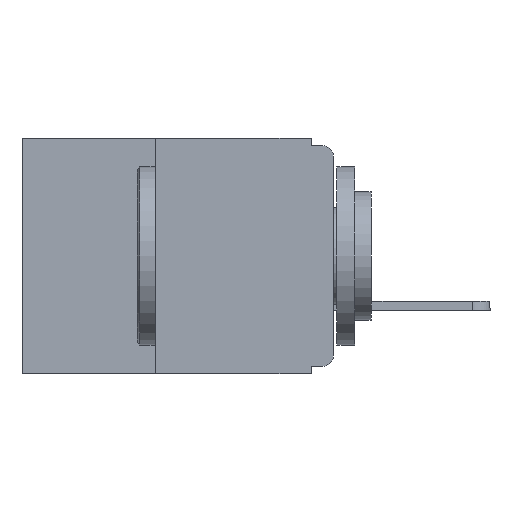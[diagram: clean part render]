
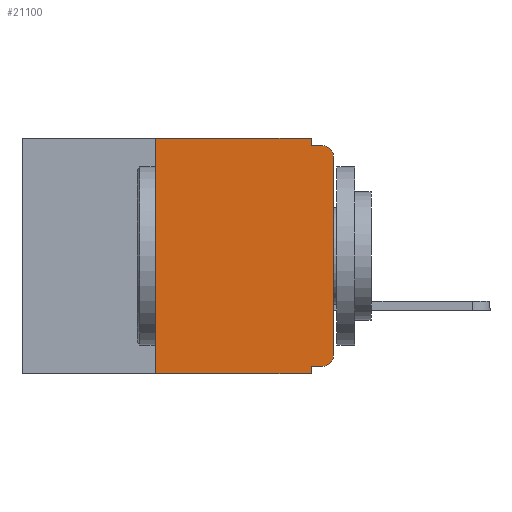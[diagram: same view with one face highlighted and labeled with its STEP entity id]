
A CAD part, left-side view. The second image highlights one B-rep face of the part: STEP entity #21100.
In plain terms, the highlighted planar face has unit normal (-1, 0, 0).
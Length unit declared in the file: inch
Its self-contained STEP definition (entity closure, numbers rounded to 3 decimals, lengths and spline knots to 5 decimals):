
#41 = VECTOR ( 'NONE', #14605, 39.37008 ) ;
#57 = DIRECTION ( 'NONE',  ( 0., -1., 0. ) ) ;
#249 = CARTESIAN_POINT ( 'NONE',  ( 0., 0., 0. ) ) ;
#356 = EDGE_CURVE ( 'NONE', #25342, #8186, #9317, .T. ) ;
#1003 = DIRECTION ( 'NONE',  ( -1., 0., 0. ) ) ;
#1020 = EDGE_CURVE ( 'NONE', #1346, #8186, #3463, .T. ) ;
#1124 = DIRECTION ( 'NONE',  ( -1., 0., 0. ) ) ;
#1240 = ORIENTED_EDGE ( 'NONE', *, *, #22163, .T. ) ;
#1346 = VERTEX_POINT ( 'NONE', #16855 ) ;
#1352 = VECTOR ( 'NONE', #9308, 39.37008 ) ;
#1428 = VERTEX_POINT ( 'NONE', #7016 ) ;
#1798 = VECTOR ( 'NONE', #15691, 39.37008 ) ;
#2524 = CARTESIAN_POINT ( 'NONE',  ( 0., 0., -0.32 ) ) ;
#3062 = PLANE ( 'NONE',  #16985 ) ;
#3365 = CARTESIAN_POINT ( 'NONE',  ( 0., 0.031, -0.33 ) ) ;
#3463 = LINE ( 'NONE', #23716, #20452 ) ;
#4282 = ORIENTED_EDGE ( 'NONE', *, *, #17504, .T. ) ;
#4568 = DIRECTION ( 'NONE',  ( 0., 1., 0. ) ) ;
#4672 = CIRCLE ( 'NONE', #18197, 0.015 ) ;
#4803 = VECTOR ( 'NONE', #22447, 39.37008 ) ;
#5467 = DIRECTION ( 'NONE',  ( 0., 0., -1. ) ) ;
#5801 = LINE ( 'NONE', #10295, #10002 ) ;
#6377 = ORIENTED_EDGE ( 'NONE', *, *, #25152, .F. ) ;
#6599 = FACE_OUTER_BOUND ( 'NONE', #18075, .T. ) ;
#6720 = CARTESIAN_POINT ( 'NONE',  ( 0., 0.25, -0.33 ) ) ;
#7016 = CARTESIAN_POINT ( 'NONE',  ( 0., 0.015, -0.32 ) ) ;
#7187 = CARTESIAN_POINT ( 'NONE',  ( 0., 0.015, -0.025 ) ) ;
#7213 = CARTESIAN_POINT ( 'NONE',  ( 0., 0.437, 0. ) ) ;
#7401 = LINE ( 'NONE', #11596, #11582 ) ;
#8174 = CARTESIAN_POINT ( 'NONE',  ( 0., 0.25, -0.33 ) ) ;
#8186 = VERTEX_POINT ( 'NONE', #26424 ) ;
#8848 = EDGE_CURVE ( 'NONE', #22550, #25099, #25296, .T. ) ;
#9159 = ORIENTED_EDGE ( 'NONE', *, *, #25471, .T. ) ;
#9291 = DIRECTION ( 'NONE',  ( 1., 0., 0. ) ) ;
#9308 = DIRECTION ( 'NONE',  ( 0., 0., -1. ) ) ;
#9317 = CIRCLE ( 'NONE', #14483, 0.015 ) ;
#9531 = VECTOR ( 'NONE', #4568, 39.37008 ) ;
#10002 = VECTOR ( 'NONE', #57, 39.37008 ) ;
#10179 = LINE ( 'NONE', #2524, #9531 ) ;
#10295 = CARTESIAN_POINT ( 'NONE',  ( 0., 0.437, -0.33 ) ) ;
#11019 = CARTESIAN_POINT ( 'NONE',  ( 0., 0.25, 0. ) ) ;
#11582 = VECTOR ( 'NONE', #5467, 39.37008 ) ;
#11596 = CARTESIAN_POINT ( 'NONE',  ( 0., 0.031, 0. ) ) ;
#11928 = EDGE_CURVE ( 'NONE', #22527, #1346, #7401, .T. ) ;
#12505 = VERTEX_POINT ( 'NONE', #3365 ) ;
#13313 = CARTESIAN_POINT ( 'NONE',  ( 0., 0.015, -0.305 ) ) ;
#14483 = AXIS2_PLACEMENT_3D ( 'NONE', #7187, #1124, #16625 ) ;
#14605 = DIRECTION ( 'NONE',  ( 0., 0., 1. ) ) ;
#14894 = EDGE_CURVE ( 'NONE', #1428, #18500, #10179, .T. ) ;
#15147 = EDGE_CURVE ( 'NONE', #25099, #22527, #23537, .T. ) ;
#15335 = DIRECTION ( 'NONE',  ( 0., 0., -1. ) ) ;
#15691 = DIRECTION ( 'NONE',  ( 0., -1., 0. ) ) ;
#16000 = CARTESIAN_POINT ( 'NONE',  ( 0., 0., -0.025 ) ) ;
#16513 = VERTEX_POINT ( 'NONE', #17197 ) ;
#16528 = ORIENTED_EDGE ( 'NONE', *, *, #1020, .F. ) ;
#16625 = DIRECTION ( 'NONE',  ( 0., 0., -1. ) ) ;
#16855 = CARTESIAN_POINT ( 'NONE',  ( 0., 0.031, -0.01 ) ) ;
#16985 = AXIS2_PLACEMENT_3D ( 'NONE', #7213, #9291, #23546 ) ;
#17197 = CARTESIAN_POINT ( 'NONE',  ( 0., 0., -0.305 ) ) ;
#17286 = ORIENTED_EDGE ( 'NONE', *, *, #8848, .F. ) ;
#17504 = EDGE_CURVE ( 'NONE', #16513, #25342, #21776, .T. ) ;
#17640 = CARTESIAN_POINT ( 'NONE',  ( 0., 0.437, 0. ) ) ;
#17663 = LINE ( 'NONE', #21421, #1352 ) ;
#17822 = CARTESIAN_POINT ( 'NONE',  ( 0., 0.031, -0.32 ) ) ;
#18075 = EDGE_LOOP ( 'NONE', ( #4282, #22678, #16528, #23976, #21176, #17286, #9159, #6377, #23751, #1240 ) ) ;
#18197 = AXIS2_PLACEMENT_3D ( 'NONE', #13313, #1003, #15335 ) ;
#18500 = VERTEX_POINT ( 'NONE', #17822 ) ;
#20452 = VECTOR ( 'NONE', #24039, 39.37008 ) ;
#21100 = ADVANCED_FACE ( 'NONE', ( #6599 ), #3062, .F. ) ;
#21176 = ORIENTED_EDGE ( 'NONE', *, *, #15147, .F. ) ;
#21421 = CARTESIAN_POINT ( 'NONE',  ( 0., 0.031, -0.33 ) ) ;
#21776 = LINE ( 'NONE', #249, #41 ) ;
#22163 = EDGE_CURVE ( 'NONE', #1428, #16513, #4672, .T. ) ;
#22447 = DIRECTION ( 'NONE',  ( 0., 0., 1. ) ) ;
#22527 = VERTEX_POINT ( 'NONE', #23051 ) ;
#22550 = VERTEX_POINT ( 'NONE', #6720 ) ;
#22678 = ORIENTED_EDGE ( 'NONE', *, *, #356, .T. ) ;
#23051 = CARTESIAN_POINT ( 'NONE',  ( 0., 0.031, 0. ) ) ;
#23537 = LINE ( 'NONE', #17640, #1798 ) ;
#23546 = DIRECTION ( 'NONE',  ( 0., 0., -1. ) ) ;
#23716 = CARTESIAN_POINT ( 'NONE',  ( 0., 0., -0.01 ) ) ;
#23751 = ORIENTED_EDGE ( 'NONE', *, *, #14894, .F. ) ;
#23976 = ORIENTED_EDGE ( 'NONE', *, *, #11928, .F. ) ;
#24039 = DIRECTION ( 'NONE',  ( 0., -1., 0. ) ) ;
#25099 = VERTEX_POINT ( 'NONE', #11019 ) ;
#25152 = EDGE_CURVE ( 'NONE', #18500, #12505, #17663, .T. ) ;
#25296 = LINE ( 'NONE', #8174, #4803 ) ;
#25342 = VERTEX_POINT ( 'NONE', #16000 ) ;
#25471 = EDGE_CURVE ( 'NONE', #22550, #12505, #5801, .T. ) ;
#26424 = CARTESIAN_POINT ( 'NONE',  ( 0., 0.015, -0.01 ) ) ;
